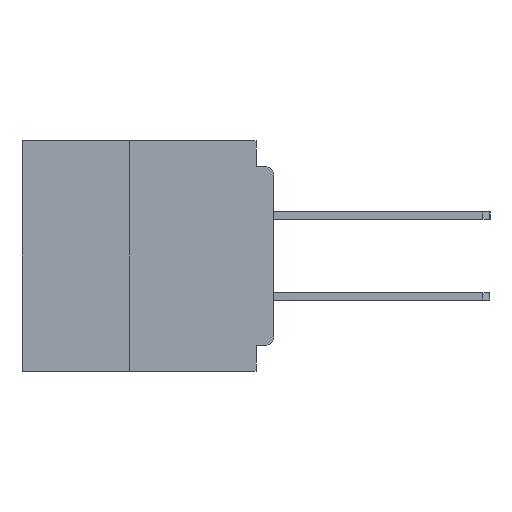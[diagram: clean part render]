
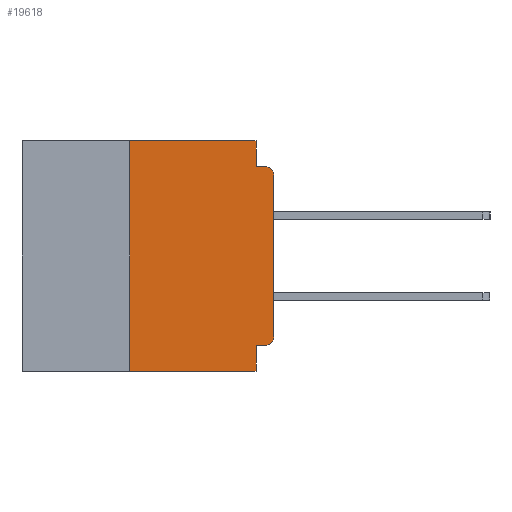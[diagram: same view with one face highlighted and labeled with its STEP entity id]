
A CAD part, left-side view. The second image highlights one B-rep face of the part: STEP entity #19618.
In plain terms, the highlighted planar face has unit normal (-1, 0, 0).
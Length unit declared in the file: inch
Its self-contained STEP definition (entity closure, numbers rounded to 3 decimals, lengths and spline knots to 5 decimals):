
#915 = DIRECTION ( 'NONE',  ( 0., 0., -1. ) ) ;
#944 = ORIENTED_EDGE ( 'NONE', *, *, #28687, .F. ) ;
#1025 = VERTEX_POINT ( 'NONE', #57628 ) ;
#1729 = CARTESIAN_POINT ( 'NONE',  ( 0., 0.031, -0.4 ) ) ;
#1885 = VERTEX_POINT ( 'NONE', #20543 ) ;
#4453 = FACE_OUTER_BOUND ( 'NONE', #5369, .T. ) ;
#4574 = DIRECTION ( 'NONE',  ( 0., -1., 0. ) ) ;
#4989 = EDGE_CURVE ( 'NONE', #6924, #44144, #16564, .T. ) ;
#5369 = EDGE_LOOP ( 'NONE', ( #60111, #9094, #944, #42776, #57833, #22422, #21453, #31278, #28656, #5387 ) ) ;
#5387 = ORIENTED_EDGE ( 'NONE', *, *, #38683, .T. ) ;
#5464 = LINE ( 'NONE', #16679, #42640 ) ;
#6568 = VERTEX_POINT ( 'NONE', #9417 ) ;
#6834 = VERTEX_POINT ( 'NONE', #1729 ) ;
#6924 = VERTEX_POINT ( 'NONE', #36346 ) ;
#6994 = LINE ( 'NONE', #10395, #44121 ) ;
#8517 = EDGE_CURVE ( 'NONE', #30157, #6568, #5464, .T. ) ;
#9094 = ORIENTED_EDGE ( 'NONE', *, *, #11997, .T. ) ;
#9417 = CARTESIAN_POINT ( 'NONE',  ( 0., 0.031, -0.045 ) ) ;
#10286 = CIRCLE ( 'NONE', #51060, 0.015 ) ;
#10387 = VERTEX_POINT ( 'NONE', #50493 ) ;
#10395 = CARTESIAN_POINT ( 'NONE',  ( 0., 0.25, -0.4 ) ) ;
#11469 = CARTESIAN_POINT ( 'NONE',  ( 0., 0., -0.355 ) ) ;
#11581 = DIRECTION ( 'NONE',  ( 0., -1., 0. ) ) ;
#11997 = EDGE_CURVE ( 'NONE', #44144, #1885, #10286, .T. ) ;
#12551 = DIRECTION ( 'NONE',  ( -1., 0., 0. ) ) ;
#13316 = CARTESIAN_POINT ( 'NONE',  ( 0., 0.437, -0.4 ) ) ;
#14431 = EDGE_CURVE ( 'NONE', #26786, #10387, #6994, .T. ) ;
#16293 = DIRECTION ( 'NONE',  ( 0., 0., -1. ) ) ;
#16564 = LINE ( 'NONE', #60196, #40747 ) ;
#16679 = CARTESIAN_POINT ( 'NONE',  ( 0., 0.031, 0. ) ) ;
#18352 = DIRECTION ( 'NONE',  ( 0., 0., -1. ) ) ;
#18738 = LINE ( 'NONE', #45202, #54248 ) ;
#19111 = CARTESIAN_POINT ( 'NONE',  ( 0., 0.437, 0. ) ) ;
#19618 = ADVANCED_FACE ( 'NONE', ( #4453 ), #40367, .F. ) ;
#20543 = CARTESIAN_POINT ( 'NONE',  ( 0., 0.015, -0.045 ) ) ;
#21453 = ORIENTED_EDGE ( 'NONE', *, *, #62337, .T. ) ;
#22422 = ORIENTED_EDGE ( 'NONE', *, *, #14431, .F. ) ;
#23561 = CIRCLE ( 'NONE', #47030, 0.015 ) ;
#24598 = LINE ( 'NONE', #13316, #50258 ) ;
#24670 = CARTESIAN_POINT ( 'NONE',  ( 0., 0., -0.06 ) ) ;
#25843 = LINE ( 'NONE', #28122, #61282 ) ;
#26786 = VERTEX_POINT ( 'NONE', #58446 ) ;
#27346 = EDGE_CURVE ( 'NONE', #10387, #30157, #46717, .T. ) ;
#28122 = CARTESIAN_POINT ( 'NONE',  ( 0., 0.031, -0.4 ) ) ;
#28656 = ORIENTED_EDGE ( 'NONE', *, *, #47245, .F. ) ;
#28687 = EDGE_CURVE ( 'NONE', #6568, #1885, #18738, .T. ) ;
#30113 = DIRECTION ( 'NONE',  ( -1., 0., 0. ) ) ;
#30157 = VERTEX_POINT ( 'NONE', #42137 ) ;
#31278 = ORIENTED_EDGE ( 'NONE', *, *, #52429, .F. ) ;
#31753 = DIRECTION ( 'NONE',  ( 0., 0., 1. ) ) ;
#32433 = VECTOR ( 'NONE', #4574, 39.37008 ) ;
#34161 = VECTOR ( 'NONE', #45297, 39.37008 ) ;
#36346 = CARTESIAN_POINT ( 'NONE',  ( 0., 0., -0.34 ) ) ;
#38683 = EDGE_CURVE ( 'NONE', #39806, #6924, #23561, .T. ) ;
#39372 = DIRECTION ( 'NONE',  ( 0., 0., 1. ) ) ;
#39806 = VERTEX_POINT ( 'NONE', #46314 ) ;
#40367 = PLANE ( 'NONE',  #43268 ) ;
#40747 = VECTOR ( 'NONE', #31753, 39.37008 ) ;
#40755 = DIRECTION ( 'NONE',  ( 0., 0., -1. ) ) ;
#41561 = CARTESIAN_POINT ( 'NONE',  ( 0., 0.015, -0.34 ) ) ;
#42137 = CARTESIAN_POINT ( 'NONE',  ( 0., 0.031, 0. ) ) ;
#42640 = VECTOR ( 'NONE', #40755, 39.37008 ) ;
#42776 = ORIENTED_EDGE ( 'NONE', *, *, #8517, .F. ) ;
#43268 = AXIS2_PLACEMENT_3D ( 'NONE', #54727, #45206, #16293 ) ;
#44121 = VECTOR ( 'NONE', #39372, 39.37008 ) ;
#44144 = VERTEX_POINT ( 'NONE', #24670 ) ;
#45202 = CARTESIAN_POINT ( 'NONE',  ( 0., 0., -0.045 ) ) ;
#45206 = DIRECTION ( 'NONE',  ( 1., 0., 0. ) ) ;
#45297 = DIRECTION ( 'NONE',  ( 0., 1., 0. ) ) ;
#46314 = CARTESIAN_POINT ( 'NONE',  ( 0., 0.015, -0.355 ) ) ;
#46358 = DIRECTION ( 'NONE',  ( 0., 0., -1. ) ) ;
#46717 = LINE ( 'NONE', #19111, #32433 ) ;
#47030 = AXIS2_PLACEMENT_3D ( 'NONE', #41561, #12551, #46358 ) ;
#47130 = DIRECTION ( 'NONE',  ( 0., -1., 0. ) ) ;
#47245 = EDGE_CURVE ( 'NONE', #39806, #1025, #56775, .T. ) ;
#50258 = VECTOR ( 'NONE', #47130, 39.37008 ) ;
#50493 = CARTESIAN_POINT ( 'NONE',  ( 0., 0.25, 0. ) ) ;
#51060 = AXIS2_PLACEMENT_3D ( 'NONE', #58973, #30113, #915 ) ;
#52429 = EDGE_CURVE ( 'NONE', #1025, #6834, #25843, .T. ) ;
#54248 = VECTOR ( 'NONE', #11581, 39.37008 ) ;
#54727 = CARTESIAN_POINT ( 'NONE',  ( 0., 0.437, 0. ) ) ;
#56775 = LINE ( 'NONE', #11469, #34161 ) ;
#57628 = CARTESIAN_POINT ( 'NONE',  ( 0., 0.031, -0.355 ) ) ;
#57833 = ORIENTED_EDGE ( 'NONE', *, *, #27346, .F. ) ;
#58446 = CARTESIAN_POINT ( 'NONE',  ( 0., 0.25, -0.4 ) ) ;
#58973 = CARTESIAN_POINT ( 'NONE',  ( 0., 0.015, -0.06 ) ) ;
#60111 = ORIENTED_EDGE ( 'NONE', *, *, #4989, .T. ) ;
#60196 = CARTESIAN_POINT ( 'NONE',  ( 0., 0., 0. ) ) ;
#61282 = VECTOR ( 'NONE', #18352, 39.37008 ) ;
#62337 = EDGE_CURVE ( 'NONE', #26786, #6834, #24598, .T. ) ;
